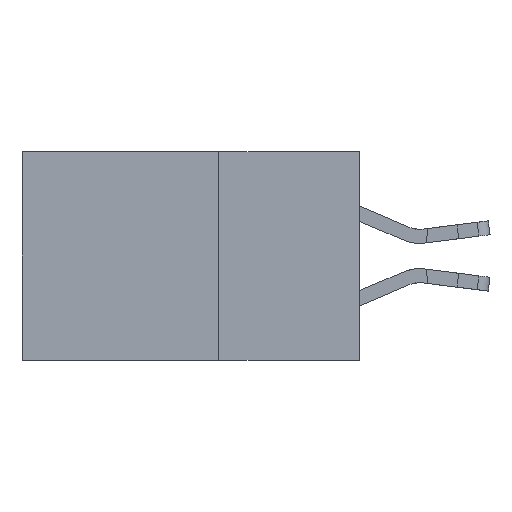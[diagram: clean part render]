
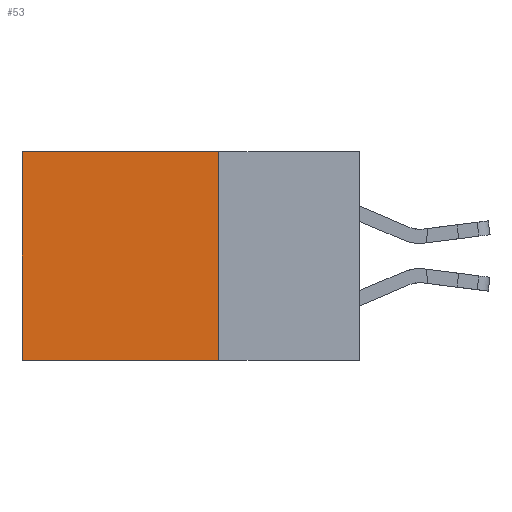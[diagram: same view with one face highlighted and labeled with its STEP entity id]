
A CAD part, left-side view. The second image highlights one B-rep face of the part: STEP entity #53.
In plain terms, the highlighted planar face has unit normal (-1, 0, 0).
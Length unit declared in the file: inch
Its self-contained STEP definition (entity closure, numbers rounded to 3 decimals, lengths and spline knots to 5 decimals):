
#53 = ADVANCED_FACE ( 'NONE', ( #8086 ), #19633, .F. ) ;
#285 = AXIS2_PLACEMENT_3D ( 'NONE', #4601, #730, #20361 ) ;
#730 = DIRECTION ( 'NONE',  ( 1., 0., 0. ) ) ;
#1271 = CARTESIAN_POINT ( 'NONE',  ( 0.2875, 0.25, 0. ) ) ;
#1313 = CARTESIAN_POINT ( 'NONE',  ( 0.2875, 0.25, -0.37 ) ) ;
#1352 = DIRECTION ( 'NONE',  ( 0., 1., 0. ) ) ;
#1572 = EDGE_CURVE ( 'NONE', #13280, #9154, #18674, .T. ) ;
#3273 = LINE ( 'NONE', #19051, #3811 ) ;
#3811 = VECTOR ( 'NONE', #9146, 39.37008 ) ;
#4518 = VECTOR ( 'NONE', #1352, 39.37008 ) ;
#4601 = CARTESIAN_POINT ( 'NONE',  ( 0.2875, 0.25, 0. ) ) ;
#6898 = EDGE_CURVE ( 'NONE', #15794, #13553, #8554, .T. ) ;
#8004 = VECTOR ( 'NONE', #18026, 39.37008 ) ;
#8086 = FACE_OUTER_BOUND ( 'NONE', #18822, .T. ) ;
#8554 = LINE ( 'NONE', #1271, #8004 ) ;
#9019 = CARTESIAN_POINT ( 'NONE',  ( 0.2875, 0.6, 0. ) ) ;
#9146 = DIRECTION ( 'NONE',  ( 0., 1., 0. ) ) ;
#9154 = VERTEX_POINT ( 'NONE', #21577 ) ;
#11123 = EDGE_CURVE ( 'NONE', #15794, #13280, #21148, .T. ) ;
#11328 = ORIENTED_EDGE ( 'NONE', *, *, #1572, .T. ) ;
#11604 = ORIENTED_EDGE ( 'NONE', *, *, #6898, .F. ) ;
#13177 = CARTESIAN_POINT ( 'NONE',  ( 0.2875, 0.25, 0. ) ) ;
#13280 = VERTEX_POINT ( 'NONE', #9019 ) ;
#13553 = VERTEX_POINT ( 'NONE', #1313 ) ;
#14339 = VECTOR ( 'NONE', #15658, 39.37008 ) ;
#15658 = DIRECTION ( 'NONE',  ( 0., 0., -1. ) ) ;
#15794 = VERTEX_POINT ( 'NONE', #18767 ) ;
#16273 = CARTESIAN_POINT ( 'NONE',  ( 0.2875, 0.6, 0. ) ) ;
#16717 = EDGE_CURVE ( 'NONE', #13553, #9154, #3273, .T. ) ;
#17461 = ORIENTED_EDGE ( 'NONE', *, *, #16717, .F. ) ;
#18026 = DIRECTION ( 'NONE',  ( 0., 0., -1. ) ) ;
#18674 = LINE ( 'NONE', #16273, #14339 ) ;
#18767 = CARTESIAN_POINT ( 'NONE',  ( 0.2875, 0.25, 0. ) ) ;
#18822 = EDGE_LOOP ( 'NONE', ( #11328, #17461, #11604, #21327 ) ) ;
#19051 = CARTESIAN_POINT ( 'NONE',  ( 0.2875, 0.25, -0.37 ) ) ;
#19633 = PLANE ( 'NONE',  #285 ) ;
#20361 = DIRECTION ( 'NONE',  ( 0., 0., -1. ) ) ;
#21148 = LINE ( 'NONE', #13177, #4518 ) ;
#21327 = ORIENTED_EDGE ( 'NONE', *, *, #11123, .T. ) ;
#21577 = CARTESIAN_POINT ( 'NONE',  ( 0.2875, 0.6, -0.37 ) ) ;
